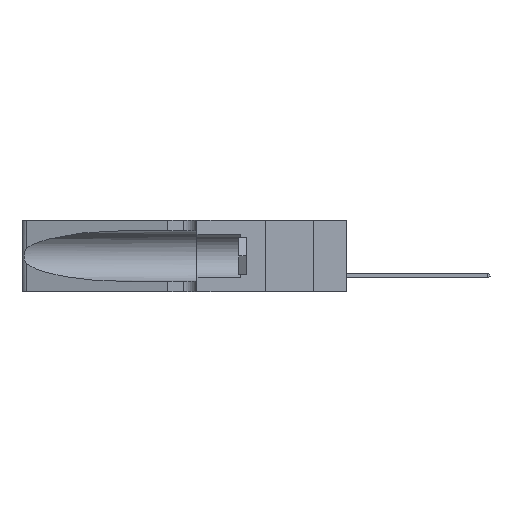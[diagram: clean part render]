
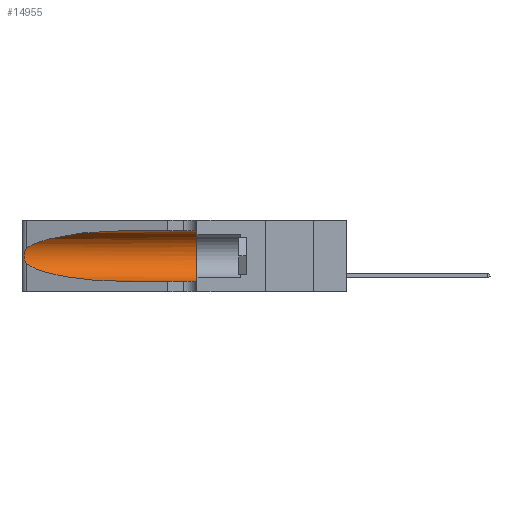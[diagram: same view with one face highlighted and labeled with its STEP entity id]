
A CAD part, left-side view. The second image highlights one B-rep face of the part: STEP entity #14955.
In plain terms, the highlighted cylindrical face has radius 3.308 mm (diameter 6.617 mm), a partial arc.
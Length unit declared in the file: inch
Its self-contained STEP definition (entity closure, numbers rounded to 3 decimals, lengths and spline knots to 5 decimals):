
#531 = EDGE_CURVE ( 'NONE', #34796, #13739, #20141, .T. ) ;
#1261 = CARTESIAN_POINT ( 'NONE',  ( 0.25787, 1.23484, 0.2124 ) ) ;
#1749 = CARTESIAN_POINT ( 'NONE',  ( 0.25854, 1.2359, 0.20912 ) ) ;
#3197 = CARTESIAN_POINT ( 'NONE',  ( 0.25487, 1.22718, 0.14631 ) ) ;
#4801 = CARTESIAN_POINT ( 'NONE',  ( 0.26018, 1.23835, 0.19895 ) ) ;
#4926 = CARTESIAN_POINT ( 'NONE',  ( 0.1305, 0.35, 0.185 ) ) ;
#5135 = CARTESIAN_POINT ( 'NONE',  ( 0.25639, 1.23186, 0.15144 ) ) ;
#5581 = VERTEX_POINT ( 'NONE', #34614 ) ;
#5853 = DIRECTION ( 'NONE',  ( 0., -1., 0. ) ) ;
#6728 = EDGE_CURVE ( 'NONE', #32969, #34144, #45540, .T. ) ;
#7238 = DIRECTION ( 'NONE',  ( 0., -1., 0. ) ) ;
#8213 = CARTESIAN_POINT ( 'NONE',  ( 0.1305, 1.61858, 0.05475 ) ) ;
#8384 = DIRECTION ( 'NONE',  ( 0., -1., 0. ) ) ;
#8392 = CARTESIAN_POINT ( 'NONE',  ( 0.26017, 1.23833, 0.17102 ) ) ;
#10587 = FACE_OUTER_BOUND ( 'NONE', #37212, .T. ) ;
#10909 = CARTESIAN_POINT ( 'NONE',  ( 0.1305, 0.35, 0.31525 ) ) ;
#11066 = CARTESIAN_POINT ( 'NONE',  ( 0.25487, 1.22718, 0.22369 ) ) ;
#11198 = CARTESIAN_POINT ( 'NONE',  ( 0.1305, 0.72297, 0.31525 ) ) ;
#11379 = CARTESIAN_POINT ( 'NONE',  ( 0.25487, 1.22718, 0.22369 ) ) ;
#11922 =( BOUNDED_CURVE ( )  B_SPLINE_CURVE ( 3, ( #3197, #20609, #45297, #31245 ),
 .UNSPECIFIED., .F., .T. ) 
 B_SPLINE_CURVE_WITH_KNOTS ( ( 4, 4 ),
 ( 3.44316, 4.71239 ),
 .UNSPECIFIED. ) 
 CURVE ( )  GEOMETRIC_REPRESENTATION_ITEM ( )  RATIONAL_B_SPLINE_CURVE ( ( 1., 0.87, 0.87, 1. ) ) 
 REPRESENTATION_ITEM ( '' )  );
#12157 = AXIS2_PLACEMENT_3D ( 'NONE', #42503, #7238, #31857 ) ;
#12370 = CARTESIAN_POINT ( 'NONE',  ( 0.25856, 1.23593, 0.16098 ) ) ;
#12489 = EDGE_CURVE ( 'NONE', #5581, #34144, #15737, .T. ) ;
#12753 = CYLINDRICAL_SURFACE ( 'NONE', #12157, 0.13025 ) ;
#13739 = VERTEX_POINT ( 'NONE', #11379 ) ;
#14759 = AXIS2_PLACEMENT_3D ( 'NONE', #4926, #23503, #38043 ) ;
#14955 = ADVANCED_FACE ( 'NONE', ( #10587 ), #12753, .F. ) ;
#15737 = LINE ( 'NONE', #8213, #21258 ) ;
#17288 = LINE ( 'NONE', #28078, #25030 ) ;
#19279 = CARTESIAN_POINT ( 'NONE',  ( 0.26075, 1.23896, 0.178 ) ) ;
#20033 = EDGE_CURVE ( 'NONE', #34796, #32969, #17288, .T. ) ;
#20141 =( BOUNDED_CURVE ( )  B_SPLINE_CURVE ( 3, ( #11198, #29080, #22004, #11066 ),
 .UNSPECIFIED., .F., .F. ) 
 B_SPLINE_CURVE_WITH_KNOTS ( ( 4, 4 ),
 ( 1.5708, 2.84003 ),
 .UNSPECIFIED. ) 
 CURVE ( )  GEOMETRIC_REPRESENTATION_ITEM ( )  RATIONAL_B_SPLINE_CURVE ( ( 1., 0.87, 0.87, 1. ) ) 
 REPRESENTATION_ITEM ( '' )  );
#20609 = CARTESIAN_POINT ( 'NONE',  ( 0.2373, 1.15595, 0.08982 ) ) ;
#20907 = ORIENTED_EDGE ( 'NONE', *, *, #12489, .T. ) ;
#21258 = VECTOR ( 'NONE', #8384, 39.37008 ) ;
#21423 = EDGE_CURVE ( 'NONE', #30088, #5581, #11922, .T. ) ;
#22004 = CARTESIAN_POINT ( 'NONE',  ( 0.2373, 1.15595, 0.28018 ) ) ;
#22630 = ORIENTED_EDGE ( 'NONE', *, *, #6728, .F. ) ;
#23503 = DIRECTION ( 'NONE',  ( 0., 1., 0. ) ) ;
#24601 = ORIENTED_EDGE ( 'NONE', *, *, #21423, .T. ) ;
#25030 = VECTOR ( 'NONE', #5853, 39.37008 ) ;
#25922 = CARTESIAN_POINT ( 'NONE',  ( 0.26075, 1.23896, 0.19203 ) ) ;
#26405 = CARTESIAN_POINT ( 'NONE',  ( 0.25487, 1.22718, 0.14631 ) ) ;
#28078 = CARTESIAN_POINT ( 'NONE',  ( 0.1305, 1.61858, 0.31525 ) ) ;
#29080 = CARTESIAN_POINT ( 'NONE',  ( 0.18966, 0.96281, 0.31525 ) ) ;
#29217 = ORIENTED_EDGE ( 'NONE', *, *, #20033, .F. ) ;
#30088 = VERTEX_POINT ( 'NONE', #33133 ) ;
#30428 = CARTESIAN_POINT ( 'NONE',  ( 0.1305, 0.35, 0.05475 ) ) ;
#30842 = CARTESIAN_POINT ( 'NONE',  ( 0.1305, 0.72297, 0.31525 ) ) ;
#31245 = CARTESIAN_POINT ( 'NONE',  ( 0.1305, 0.72297, 0.05475 ) ) ;
#31337 = ORIENTED_EDGE ( 'NONE', *, *, #41357, .T. ) ;
#31857 = DIRECTION ( 'NONE',  ( 0., 0., -1. ) ) ;
#32858 = CARTESIAN_POINT ( 'NONE',  ( 0.25487, 1.22718, 0.22369 ) ) ;
#32969 = VERTEX_POINT ( 'NONE', #10909 ) ;
#33133 = CARTESIAN_POINT ( 'NONE',  ( 0.25487, 1.22718, 0.14631 ) ) ;
#33182 = CARTESIAN_POINT ( 'NONE',  ( 0.25789, 1.23486, 0.15765 ) ) ;
#34144 = VERTEX_POINT ( 'NONE', #30428 ) ;
#34614 = CARTESIAN_POINT ( 'NONE',  ( 0.1305, 0.72297, 0.05475 ) ) ;
#34796 = VERTEX_POINT ( 'NONE', #30842 ) ;
#37078 = B_SPLINE_CURVE_WITH_KNOTS ( 'NONE', 3,
 ( #32858, #40438, #43841, #1261, #1749, #4801, #25922, #19279, #8392, #12370, #33182, #5135, #44148, #26405 ),
 .UNSPECIFIED., .F., .F.,
 ( 4, 2, 2, 2, 2, 2, 4 ),
 ( 0., 0.00027, 0.00053, 0.00107, 0.0016, 0.00187, 0.00214 ),
 .UNSPECIFIED. ) ;
#37212 = EDGE_LOOP ( 'NONE', ( #38829, #31337, #24601, #20907, #22630, #29217 ) ) ;
#38043 = DIRECTION ( 'NONE',  ( 0., 0., 1. ) ) ;
#38829 = ORIENTED_EDGE ( 'NONE', *, *, #531, .T. ) ;
#40438 = CARTESIAN_POINT ( 'NONE',  ( 0.25555, 1.22994, 0.2215 ) ) ;
#41357 = EDGE_CURVE ( 'NONE', #13739, #30088, #37078, .T. ) ;
#42503 = CARTESIAN_POINT ( 'NONE',  ( 0.1305, 1.61858, 0.185 ) ) ;
#43841 = CARTESIAN_POINT ( 'NONE',  ( 0.25639, 1.23184, 0.21858 ) ) ;
#44148 = CARTESIAN_POINT ( 'NONE',  ( 0.25555, 1.22993, 0.14849 ) ) ;
#45297 = CARTESIAN_POINT ( 'NONE',  ( 0.18966, 0.96281, 0.05475 ) ) ;
#45540 = CIRCLE ( 'NONE', #14759, 0.13025 ) ;
